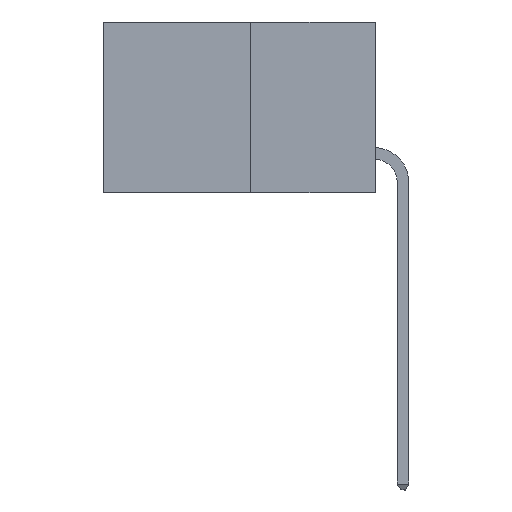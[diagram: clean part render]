
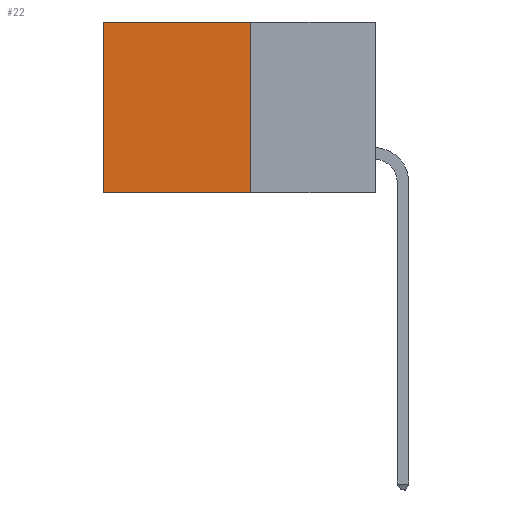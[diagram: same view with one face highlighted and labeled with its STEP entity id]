
A CAD part, left-side view. The second image highlights one B-rep face of the part: STEP entity #22.
In plain terms, the highlighted planar face has unit normal (-1, 0, 0).
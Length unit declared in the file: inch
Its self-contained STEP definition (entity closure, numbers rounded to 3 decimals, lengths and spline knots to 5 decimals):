
#22 = ADVANCED_FACE ( 'NONE', ( #7986 ), #19045, .F. ) ;
#958 = VECTOR ( 'NONE', #12674, 39.37008 ) ;
#2232 = LINE ( 'NONE', #13034, #26051 ) ;
#2266 = ORIENTED_EDGE ( 'NONE', *, *, #7221, .F. ) ;
#3282 = CARTESIAN_POINT ( 'NONE',  ( 0.277, 0.27, -0.37 ) ) ;
#3588 = VECTOR ( 'NONE', #18951, 39.37008 ) ;
#3833 = VERTEX_POINT ( 'NONE', #13752 ) ;
#3957 = EDGE_LOOP ( 'NONE', ( #12749, #24318, #2266, #24417 ) ) ;
#4221 = VERTEX_POINT ( 'NONE', #17138 ) ;
#5558 = EDGE_CURVE ( 'NONE', #3833, #14149, #6878, .T. ) ;
#5797 = VERTEX_POINT ( 'NONE', #13452 ) ;
#6532 = CARTESIAN_POINT ( 'NONE',  ( 0.277, 0.59, -0.37 ) ) ;
#6878 = LINE ( 'NONE', #17168, #958 ) ;
#7221 = EDGE_CURVE ( 'NONE', #4221, #5797, #2232, .T. ) ;
#7652 = EDGE_CURVE ( 'NONE', #5797, #14149, #20056, .T. ) ;
#7671 = EDGE_CURVE ( 'NONE', #4221, #3833, #25322, .T. ) ;
#7986 = FACE_OUTER_BOUND ( 'NONE', #3957, .T. ) ;
#8183 = CARTESIAN_POINT ( 'NONE',  ( 0.277, 0.27, -0.37 ) ) ;
#10083 = DIRECTION ( 'NONE',  ( 0., 1., 0. ) ) ;
#11839 = AXIS2_PLACEMENT_3D ( 'NONE', #8183, #22064, #21417 ) ;
#12674 = DIRECTION ( 'NONE',  ( 0., 0., -1. ) ) ;
#12749 = ORIENTED_EDGE ( 'NONE', *, *, #5558, .T. ) ;
#13034 = CARTESIAN_POINT ( 'NONE',  ( 0.277, 0.27, -0.37 ) ) ;
#13452 = CARTESIAN_POINT ( 'NONE',  ( 0.277, 0.27, -0.37 ) ) ;
#13752 = CARTESIAN_POINT ( 'NONE',  ( 0.277, 0.59, 0. ) ) ;
#14149 = VERTEX_POINT ( 'NONE', #6532 ) ;
#17138 = CARTESIAN_POINT ( 'NONE',  ( 0.277, 0.27, 0. ) ) ;
#17168 = CARTESIAN_POINT ( 'NONE',  ( 0.277, 0.59, -0.37 ) ) ;
#18951 = DIRECTION ( 'NONE',  ( 0., 1., 0. ) ) ;
#19045 = PLANE ( 'NONE',  #11839 ) ;
#19353 = VECTOR ( 'NONE', #10083, 39.37008 ) ;
#20056 = LINE ( 'NONE', #3282, #3588 ) ;
#21417 = DIRECTION ( 'NONE',  ( 0., 0., -1. ) ) ;
#22064 = DIRECTION ( 'NONE',  ( 1., 0., 0. ) ) ;
#24318 = ORIENTED_EDGE ( 'NONE', *, *, #7652, .F. ) ;
#24417 = ORIENTED_EDGE ( 'NONE', *, *, #7671, .T. ) ;
#25322 = LINE ( 'NONE', #25727, #19353 ) ;
#25727 = CARTESIAN_POINT ( 'NONE',  ( 0.277, 0.27, 0. ) ) ;
#26051 = VECTOR ( 'NONE', #28691, 39.37008 ) ;
#28691 = DIRECTION ( 'NONE',  ( 0., 0., -1. ) ) ;
